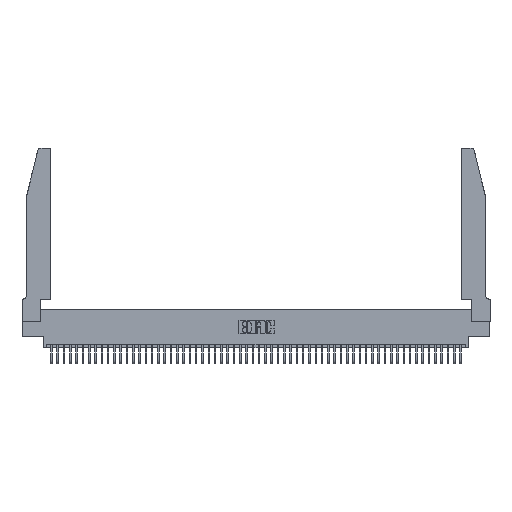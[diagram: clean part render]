
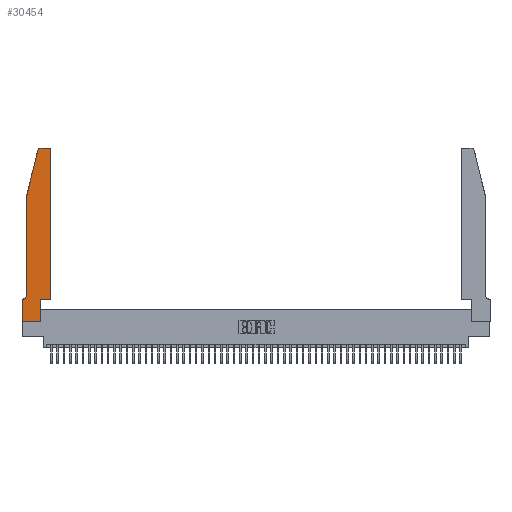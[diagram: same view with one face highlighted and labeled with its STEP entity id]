
A CAD part, top view. The second image highlights one B-rep face of the part: STEP entity #30454.
In plain terms, the highlighted planar face has unit normal (0, 0, 1).
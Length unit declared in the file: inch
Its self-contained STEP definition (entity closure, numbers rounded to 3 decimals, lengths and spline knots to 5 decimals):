
#614 = VERTEX_POINT ( 'NONE', #41289 ) ;
#1278 = LINE ( 'NONE', #28515, #41041 ) ;
#1706 = ORIENTED_EDGE ( 'NONE', *, *, #1815, .T. ) ;
#1747 = ORIENTED_EDGE ( 'NONE', *, *, #46496, .T. ) ;
#1815 = EDGE_CURVE ( 'NONE', #32682, #614, #41472, .T. ) ;
#2041 = DIRECTION ( 'NONE',  ( -1., 0., 0. ) ) ;
#2678 = LINE ( 'NONE', #21832, #13232 ) ;
#2827 = CIRCLE ( 'NONE', #47358, 0.03 ) ;
#2854 = EDGE_CURVE ( 'NONE', #24790, #45678, #1278, .T. ) ;
#2885 = CARTESIAN_POINT ( 'NONE',  ( 0.4505, 0.35, 0.37 ) ) ;
#4553 = CARTESIAN_POINT ( 'NONE',  ( 0.25487, 2.72718, 0.37 ) ) ;
#4586 = DIRECTION ( 'NONE',  ( 0., -1., 0. ) ) ;
#5448 = ORIENTED_EDGE ( 'NONE', *, *, #18372, .T. ) ;
#5676 = DIRECTION ( 'NONE',  ( 1., 0., 0. ) ) ;
#5811 = DIRECTION ( 'NONE',  ( 1., 0., 0. ) ) ;
#6530 = LINE ( 'NONE', #16527, #26352 ) ;
#7537 = CARTESIAN_POINT ( 'NONE',  ( 0.0055, 0.42, 0.37 ) ) ;
#7783 = LINE ( 'NONE', #2885, #38194 ) ;
#8312 = DIRECTION ( 'NONE',  ( 0., 0., 1. ) ) ;
#9595 = CARTESIAN_POINT ( 'NONE',  ( 0.284, 2.75, 0.37 ) ) ;
#9610 = CARTESIAN_POINT ( 'NONE',  ( 0.2865, 0.35, 0.37 ) ) ;
#10031 = VECTOR ( 'NONE', #27749, 39.37008 ) ;
#10400 = ORIENTED_EDGE ( 'NONE', *, *, #11057, .T. ) ;
#10528 = CARTESIAN_POINT ( 'NONE',  ( 0.0755, 0.42, 0.37 ) ) ;
#11057 = EDGE_CURVE ( 'NONE', #614, #13172, #40131, .T. ) ;
#11522 = DIRECTION ( 'NONE',  ( -1., 0., 0. ) ) ;
#12945 = ORIENTED_EDGE ( 'NONE', *, *, #2854, .T. ) ;
#13172 = VERTEX_POINT ( 'NONE', #10528 ) ;
#13232 = VECTOR ( 'NONE', #2041, 39.37008 ) ;
#13688 = DIRECTION ( 'NONE',  ( -0.239, -0.971, 0. ) ) ;
#14752 = ORIENTED_EDGE ( 'NONE', *, *, #16541, .T. ) ;
#16076 = CARTESIAN_POINT ( 'NONE',  ( 0.4505, 2.72, 0.37 ) ) ;
#16527 = CARTESIAN_POINT ( 'NONE',  ( 0.2865, 0.35, 0.37 ) ) ;
#16541 = EDGE_CURVE ( 'NONE', #21939, #24790, #2678, .T. ) ;
#17677 = VERTEX_POINT ( 'NONE', #48965 ) ;
#18101 = DIRECTION ( 'NONE',  ( 0., 0., 1. ) ) ;
#18372 = EDGE_CURVE ( 'NONE', #45678, #22535, #32943, .T. ) ;
#19138 = AXIS2_PLACEMENT_3D ( 'NONE', #7537, #35295, #11522 ) ;
#20345 = CARTESIAN_POINT ( 'NONE',  ( 0.0755, 2., 0.37 ) ) ;
#21832 = CARTESIAN_POINT ( 'NONE',  ( 0.0755, 0.35, 0.37 ) ) ;
#21939 = VERTEX_POINT ( 'NONE', #22254 ) ;
#22157 = EDGE_CURVE ( 'NONE', #22535, #40945, #6530, .T. ) ;
#22254 = CARTESIAN_POINT ( 'NONE',  ( 0.0055, 0.35, 0.37 ) ) ;
#22535 = VERTEX_POINT ( 'NONE', #34692 ) ;
#22977 = LINE ( 'NONE', #26647, #32328 ) ;
#24681 = ORIENTED_EDGE ( 'NONE', *, *, #25205, .T. ) ;
#24790 = VERTEX_POINT ( 'NONE', #36740 ) ;
#25205 = EDGE_CURVE ( 'NONE', #13172, #21939, #38565, .T. ) ;
#25562 = CARTESIAN_POINT ( 'NONE',  ( 0., 0.35, 0.37 ) ) ;
#26207 = CARTESIAN_POINT ( 'NONE',  ( 0., 0., 0.37 ) ) ;
#26352 = VECTOR ( 'NONE', #36487, 39.37008 ) ;
#26647 = CARTESIAN_POINT ( 'NONE',  ( 0.4505, 0.35, 0.37 ) ) ;
#27749 = DIRECTION ( 'NONE',  ( -1., 0., 0. ) ) ;
#27760 = CIRCLE ( 'NONE', #46892, 0.03 ) ;
#28131 = DIRECTION ( 'NONE',  ( 0., -1., 0. ) ) ;
#28147 = EDGE_CURVE ( 'NONE', #17677, #49314, #22977, .T. ) ;
#28515 = CARTESIAN_POINT ( 'NONE',  ( 0., 0., 0.37 ) ) ;
#29503 = CARTESIAN_POINT ( 'NONE',  ( 0.0755, 2., 0.37 ) ) ;
#29587 = DIRECTION ( 'NONE',  ( 0., 0., 1. ) ) ;
#30454 = ADVANCED_FACE ( 'NONE', ( #51353 ), #49342, .T. ) ;
#30530 = EDGE_CURVE ( 'NONE', #43245, #32682, #27760, .T. ) ;
#30770 = EDGE_LOOP ( 'NONE', ( #37063, #44587, #1706, #10400, #24681, #14752, #12945, #5448, #39577, #43351, #47061, #1747 ) ) ;
#30879 = VECTOR ( 'NONE', #13688, 39.37008 ) ;
#31853 = EDGE_CURVE ( 'NONE', #40945, #17677, #7783, .T. ) ;
#32099 = CARTESIAN_POINT ( 'NONE',  ( 0.4205, 2.72, 0.37 ) ) ;
#32328 = VECTOR ( 'NONE', #38497, 39.37008 ) ;
#32682 = VERTEX_POINT ( 'NONE', #4553 ) ;
#32943 = LINE ( 'NONE', #33434, #42251 ) ;
#33434 = CARTESIAN_POINT ( 'NONE',  ( 0., 0., 0.37 ) ) ;
#34453 = DIRECTION ( 'NONE',  ( 1., 0., 0. ) ) ;
#34692 = CARTESIAN_POINT ( 'NONE',  ( 0.2865, 0., 0.37 ) ) ;
#35295 = DIRECTION ( 'NONE',  ( 0., 0., -1. ) ) ;
#36085 = DIRECTION ( 'NONE',  ( 1., 0., 0. ) ) ;
#36487 = DIRECTION ( 'NONE',  ( 0., 1., 0. ) ) ;
#36740 = CARTESIAN_POINT ( 'NONE',  ( 0., 0.35, 0.37 ) ) ;
#37063 = ORIENTED_EDGE ( 'NONE', *, *, #39356, .T. ) ;
#38194 = VECTOR ( 'NONE', #34453, 39.37008 ) ;
#38497 = DIRECTION ( 'NONE',  ( 0., 1., 0. ) ) ;
#38565 = CIRCLE ( 'NONE', #19138, 0.07 ) ;
#38900 = AXIS2_PLACEMENT_3D ( 'NONE', #25562, #29587, #5811 ) ;
#39356 = EDGE_CURVE ( 'NONE', #48407, #43245, #41739, .T. ) ;
#39577 = ORIENTED_EDGE ( 'NONE', *, *, #22157, .T. ) ;
#40131 = LINE ( 'NONE', #20345, #49435 ) ;
#40945 = VERTEX_POINT ( 'NONE', #9610 ) ;
#41041 = VECTOR ( 'NONE', #4586, 39.37008 ) ;
#41289 = CARTESIAN_POINT ( 'NONE',  ( 0.0755, 2., 0.37 ) ) ;
#41472 = LINE ( 'NONE', #29503, #30879 ) ;
#41739 = LINE ( 'NONE', #43628, #10031 ) ;
#41908 = CARTESIAN_POINT ( 'NONE',  ( 0.284, 2.72, 0.37 ) ) ;
#42251 = VECTOR ( 'NONE', #5676, 39.37008 ) ;
#43245 = VERTEX_POINT ( 'NONE', #9595 ) ;
#43351 = ORIENTED_EDGE ( 'NONE', *, *, #31853, .T. ) ;
#43628 = CARTESIAN_POINT ( 'NONE',  ( 0.2605, 2.75, 0.37 ) ) ;
#44587 = ORIENTED_EDGE ( 'NONE', *, *, #30530, .T. ) ;
#45678 = VERTEX_POINT ( 'NONE', #26207 ) ;
#45894 = DIRECTION ( 'NONE',  ( 1., 0., 0. ) ) ;
#46496 = EDGE_CURVE ( 'NONE', #49314, #48407, #2827, .T. ) ;
#46892 = AXIS2_PLACEMENT_3D ( 'NONE', #41908, #18101, #45894 ) ;
#47061 = ORIENTED_EDGE ( 'NONE', *, *, #28147, .T. ) ;
#47358 = AXIS2_PLACEMENT_3D ( 'NONE', #32099, #8312, #36085 ) ;
#48407 = VERTEX_POINT ( 'NONE', #50139 ) ;
#48965 = CARTESIAN_POINT ( 'NONE',  ( 0.4505, 0.35, 0.37 ) ) ;
#49314 = VERTEX_POINT ( 'NONE', #16076 ) ;
#49342 = PLANE ( 'NONE',  #38900 ) ;
#49435 = VECTOR ( 'NONE', #28131, 39.37008 ) ;
#50139 = CARTESIAN_POINT ( 'NONE',  ( 0.4205, 2.75, 0.37 ) ) ;
#51353 = FACE_OUTER_BOUND ( 'NONE', #30770, .T. ) ;
